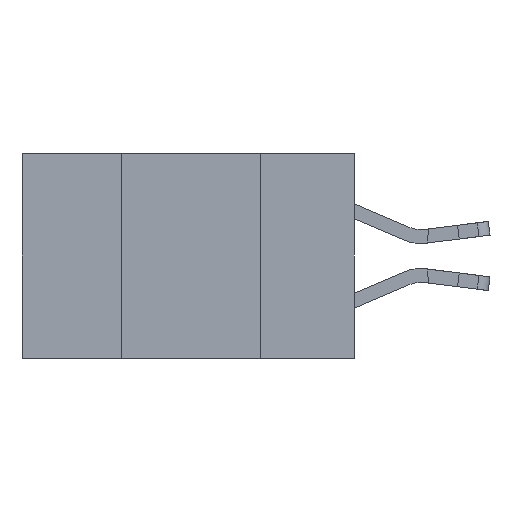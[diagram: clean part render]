
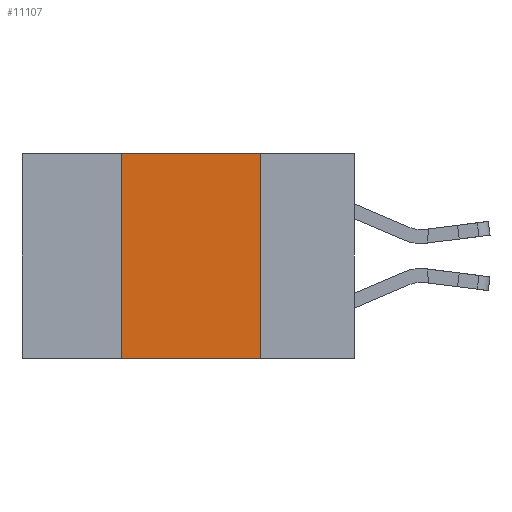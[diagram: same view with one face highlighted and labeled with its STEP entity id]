
A CAD part, left-side view. The second image highlights one B-rep face of the part: STEP entity #11107.
In plain terms, the highlighted planar face has unit normal (-1, 0, 0).
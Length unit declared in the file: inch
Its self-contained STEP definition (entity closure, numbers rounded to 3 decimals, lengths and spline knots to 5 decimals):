
#127 = DIRECTION ( 'NONE',  ( 0., 0., -1. ) ) ;
#380 = CARTESIAN_POINT ( 'NONE',  ( 0., 0.17, 0. ) ) ;
#505 = CARTESIAN_POINT ( 'NONE',  ( 0., 0.17, -0.37 ) ) ;
#1595 = VECTOR ( 'NONE', #19635, 39.37008 ) ;
#2039 = CARTESIAN_POINT ( 'NONE',  ( 0., 0.42, -0.37 ) ) ;
#2692 = VECTOR ( 'NONE', #16140, 39.37008 ) ;
#2886 = ORIENTED_EDGE ( 'NONE', *, *, #16109, .F. ) ;
#3108 = LINE ( 'NONE', #10233, #11542 ) ;
#5823 = CARTESIAN_POINT ( 'NONE',  ( 0., 0.6, 0. ) ) ;
#6357 = CARTESIAN_POINT ( 'NONE',  ( 0., 0.42, -0.37 ) ) ;
#6594 = LINE ( 'NONE', #6357, #19466 ) ;
#6951 = EDGE_LOOP ( 'NONE', ( #14012, #2886, #11193, #9233 ) ) ;
#7589 = FACE_OUTER_BOUND ( 'NONE', #6951, .T. ) ;
#8793 = LINE ( 'NONE', #15690, #2692 ) ;
#9110 = PLANE ( 'NONE',  #11672 ) ;
#9233 = ORIENTED_EDGE ( 'NONE', *, *, #20541, .T. ) ;
#9505 = VERTEX_POINT ( 'NONE', #18771 ) ;
#10233 = CARTESIAN_POINT ( 'NONE',  ( 0., 0.6, 0. ) ) ;
#10371 = EDGE_CURVE ( 'NONE', #17548, #9505, #6594, .T. ) ;
#10696 = EDGE_CURVE ( 'NONE', #22672, #14420, #14379, .T. ) ;
#11107 = ADVANCED_FACE ( 'NONE', ( #7589 ), #9110, .F. ) ;
#11193 = ORIENTED_EDGE ( 'NONE', *, *, #10371, .F. ) ;
#11542 = VECTOR ( 'NONE', #18970, 39.37008 ) ;
#11672 = AXIS2_PLACEMENT_3D ( 'NONE', #5823, #12952, #127 ) ;
#12952 = DIRECTION ( 'NONE',  ( 1., 0., 0. ) ) ;
#13601 = DIRECTION ( 'NONE',  ( 0., 0., 1. ) ) ;
#14012 = ORIENTED_EDGE ( 'NONE', *, *, #10696, .F. ) ;
#14379 = LINE ( 'NONE', #16598, #1595 ) ;
#14420 = VERTEX_POINT ( 'NONE', #505 ) ;
#15690 = CARTESIAN_POINT ( 'NONE',  ( 0., 0.6, -0.37 ) ) ;
#16109 = EDGE_CURVE ( 'NONE', #9505, #22672, #3108, .T. ) ;
#16140 = DIRECTION ( 'NONE',  ( 0., -1., 0. ) ) ;
#16598 = CARTESIAN_POINT ( 'NONE',  ( 0., 0.17, -0.37 ) ) ;
#17548 = VERTEX_POINT ( 'NONE', #2039 ) ;
#18771 = CARTESIAN_POINT ( 'NONE',  ( 0., 0.42, 0. ) ) ;
#18970 = DIRECTION ( 'NONE',  ( 0., -1., 0. ) ) ;
#19466 = VECTOR ( 'NONE', #13601, 39.37008 ) ;
#19635 = DIRECTION ( 'NONE',  ( 0., 0., -1. ) ) ;
#20541 = EDGE_CURVE ( 'NONE', #17548, #14420, #8793, .T. ) ;
#22672 = VERTEX_POINT ( 'NONE', #380 ) ;
